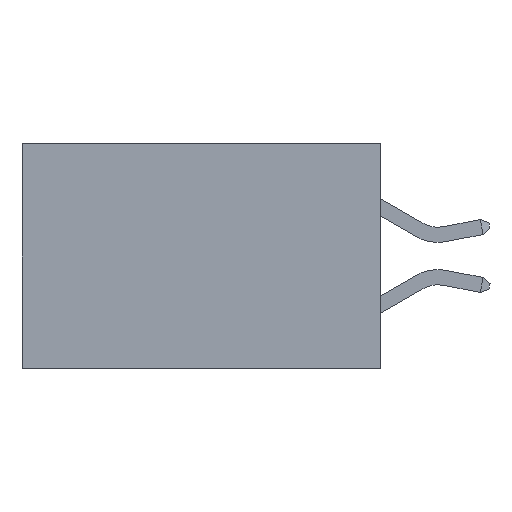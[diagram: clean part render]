
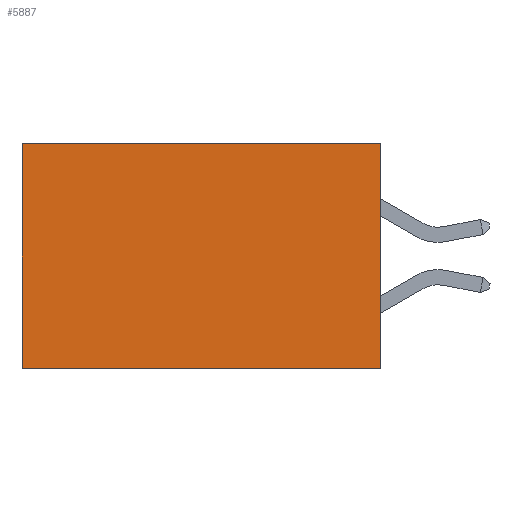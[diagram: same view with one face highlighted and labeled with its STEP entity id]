
A CAD part, left-side view. The second image highlights one B-rep face of the part: STEP entity #5887.
In plain terms, the highlighted planar face has unit normal (-1, 0, 0).
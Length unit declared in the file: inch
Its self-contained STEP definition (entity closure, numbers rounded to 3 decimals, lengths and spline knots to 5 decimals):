
#1640 = LINE ( 'NONE', #21554, #21169 ) ;
#1704 = ORIENTED_EDGE ( 'NONE', *, *, #17540, .T. ) ;
#1872 = CARTESIAN_POINT ( 'NONE',  ( 0.277, 0., 0. ) ) ;
#2554 = AXIS2_PLACEMENT_3D ( 'NONE', #13705, #28123, #12074 ) ;
#3642 = ORIENTED_EDGE ( 'NONE', *, *, #26554, .F. ) ;
#3970 = ORIENTED_EDGE ( 'NONE', *, *, #23319, .T. ) ;
#4693 = DIRECTION ( 'NONE',  ( 0., 1., 0. ) ) ;
#5887 = ADVANCED_FACE ( 'NONE', ( #17237 ), #12336, .F. ) ;
#7040 = VECTOR ( 'NONE', #12776, 39.37008 ) ;
#7834 = LINE ( 'NONE', #20485, #7040 ) ;
#8488 = CARTESIAN_POINT ( 'NONE',  ( 0.277, 0.59, -0.37 ) ) ;
#8575 = DIRECTION ( 'NONE',  ( 0., 0., -1. ) ) ;
#9102 = VERTEX_POINT ( 'NONE', #29589 ) ;
#9787 = CARTESIAN_POINT ( 'NONE',  ( 0.277, 0., 0. ) ) ;
#12074 = DIRECTION ( 'NONE',  ( 0., 0., -1. ) ) ;
#12336 = PLANE ( 'NONE',  #2554 ) ;
#12776 = DIRECTION ( 'NONE',  ( 0., 1., 0. ) ) ;
#13705 = CARTESIAN_POINT ( 'NONE',  ( 0.277, 0., -0.37 ) ) ;
#15366 = LINE ( 'NONE', #23838, #28994 ) ;
#17237 = FACE_OUTER_BOUND ( 'NONE', #29197, .T. ) ;
#17540 = EDGE_CURVE ( 'NONE', #22336, #27887, #15366, .T. ) ;
#18770 = VERTEX_POINT ( 'NONE', #1872 ) ;
#20485 = CARTESIAN_POINT ( 'NONE',  ( 0.277, 0., -0.37 ) ) ;
#21169 = VECTOR ( 'NONE', #24148, 39.37008 ) ;
#21554 = CARTESIAN_POINT ( 'NONE',  ( 0.277, 0., -0.37 ) ) ;
#22336 = VERTEX_POINT ( 'NONE', #31909 ) ;
#23319 = EDGE_CURVE ( 'NONE', #18770, #22336, #24151, .T. ) ;
#23838 = CARTESIAN_POINT ( 'NONE',  ( 0.277, 0.59, -0.37 ) ) ;
#24148 = DIRECTION ( 'NONE',  ( 0., 0., -1. ) ) ;
#24151 = LINE ( 'NONE', #9787, #30932 ) ;
#26554 = EDGE_CURVE ( 'NONE', #18770, #9102, #1640, .T. ) ;
#27139 = ORIENTED_EDGE ( 'NONE', *, *, #28569, .F. ) ;
#27887 = VERTEX_POINT ( 'NONE', #8488 ) ;
#28123 = DIRECTION ( 'NONE',  ( 1., 0., 0. ) ) ;
#28569 = EDGE_CURVE ( 'NONE', #9102, #27887, #7834, .T. ) ;
#28994 = VECTOR ( 'NONE', #8575, 39.37008 ) ;
#29197 = EDGE_LOOP ( 'NONE', ( #1704, #27139, #3642, #3970 ) ) ;
#29589 = CARTESIAN_POINT ( 'NONE',  ( 0.277, 0., -0.37 ) ) ;
#30932 = VECTOR ( 'NONE', #4693, 39.37008 ) ;
#31909 = CARTESIAN_POINT ( 'NONE',  ( 0.277, 0.59, 0. ) ) ;
